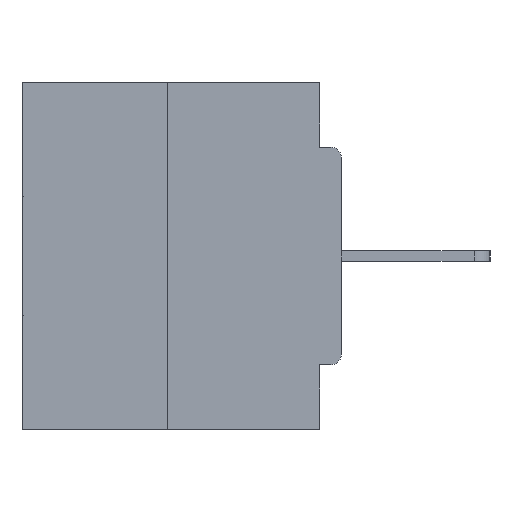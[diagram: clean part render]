
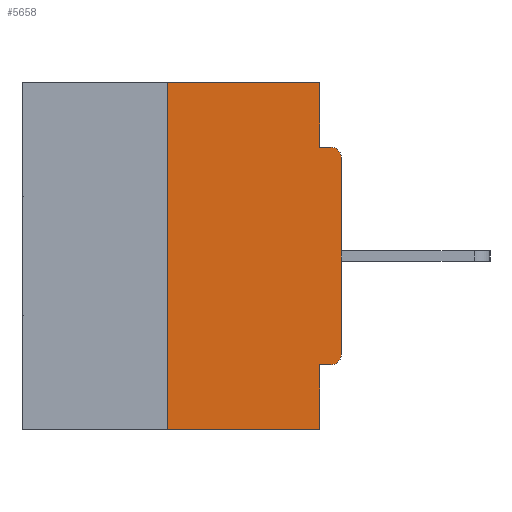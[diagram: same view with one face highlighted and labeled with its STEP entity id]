
A CAD part, left-side view. The second image highlights one B-rep face of the part: STEP entity #5658.
In plain terms, the highlighted planar face has unit normal (-1, 0, 0).
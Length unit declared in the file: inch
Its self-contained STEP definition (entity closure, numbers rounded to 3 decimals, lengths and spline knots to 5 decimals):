
#301 = LINE ( 'NONE', #3106, #26805 ) ;
#2354 = ORIENTED_EDGE ( 'NONE', *, *, #10486, .F. ) ;
#2415 = CARTESIAN_POINT ( 'NONE',  ( 0., 0., -0.4065 ) ) ;
#2515 = EDGE_CURVE ( 'NONE', #10941, #27300, #4757, .T. ) ;
#2608 = DIRECTION ( 'NONE',  ( 0., -1., 0. ) ) ;
#2764 = VECTOR ( 'NONE', #17830, 39.37008 ) ;
#2920 = EDGE_CURVE ( 'NONE', #7568, #13568, #19948, .T. ) ;
#3105 = ORIENTED_EDGE ( 'NONE', *, *, #10581, .F. ) ;
#3106 = CARTESIAN_POINT ( 'NONE',  ( 0., 0.46, 0. ) ) ;
#3801 = LINE ( 'NONE', #24804, #9874 ) ;
#4358 = DIRECTION ( 'NONE',  ( 0., 0., -1. ) ) ;
#4757 = CIRCLE ( 'NONE', #12188, 0.015 ) ;
#5425 = VECTOR ( 'NONE', #16728, 39.37008 ) ;
#5658 = ADVANCED_FACE ( 'NONE', ( #11987 ), #13768, .F. ) ;
#6357 = VECTOR ( 'NONE', #24160, 39.37008 ) ;
#6729 = CARTESIAN_POINT ( 'NONE',  ( 0., 0.015, -0.1085 ) ) ;
#7568 = VERTEX_POINT ( 'NONE', #27094 ) ;
#8507 = ORIENTED_EDGE ( 'NONE', *, *, #2515, .T. ) ;
#9056 = EDGE_CURVE ( 'NONE', #9649, #16005, #301, .T. ) ;
#9332 = DIRECTION ( 'NONE',  ( 0., 0., -1. ) ) ;
#9472 = DIRECTION ( 'NONE',  ( 0., -1., 0. ) ) ;
#9649 = VERTEX_POINT ( 'NONE', #28711 ) ;
#9679 = LINE ( 'NONE', #2415, #2764 ) ;
#9694 = CARTESIAN_POINT ( 'NONE',  ( 0., 0., -0.3915 ) ) ;
#9874 = VECTOR ( 'NONE', #4358, 39.37008 ) ;
#10486 = EDGE_CURVE ( 'NONE', #22350, #28929, #13092, .T. ) ;
#10581 = EDGE_CURVE ( 'NONE', #16005, #22350, #3801, .T. ) ;
#10941 = VERTEX_POINT ( 'NONE', #26113 ) ;
#11171 = CIRCLE ( 'NONE', #15982, 0.015 ) ;
#11987 = FACE_OUTER_BOUND ( 'NONE', #19914, .T. ) ;
#12012 = VERTEX_POINT ( 'NONE', #26157 ) ;
#12188 = AXIS2_PLACEMENT_3D ( 'NONE', #31875, #31736, #31626 ) ;
#12704 = DIRECTION ( 'NONE',  ( 0., 0., -1. ) ) ;
#12757 = LINE ( 'NONE', #19591, #18703 ) ;
#13043 = ORIENTED_EDGE ( 'NONE', *, *, #25138, .F. ) ;
#13092 = LINE ( 'NONE', #19384, #5425 ) ;
#13142 = DIRECTION ( 'NONE',  ( 1., 0., 0. ) ) ;
#13568 = VERTEX_POINT ( 'NONE', #16201 ) ;
#13600 = EDGE_CURVE ( 'NONE', #27300, #22740, #17678, .T. ) ;
#13768 = PLANE ( 'NONE',  #20550 ) ;
#14583 = CARTESIAN_POINT ( 'NONE',  ( 0., 0.46, 0. ) ) ;
#15982 = AXIS2_PLACEMENT_3D ( 'NONE', #6729, #24567, #9332 ) ;
#16005 = VERTEX_POINT ( 'NONE', #16865 ) ;
#16201 = CARTESIAN_POINT ( 'NONE',  ( 0., 0.031, -0.5 ) ) ;
#16315 = CARTESIAN_POINT ( 'NONE',  ( 0., 0., 0. ) ) ;
#16681 = EDGE_CURVE ( 'NONE', #12012, #13568, #12757, .T. ) ;
#16728 = DIRECTION ( 'NONE',  ( 0., -1., 0. ) ) ;
#16865 = CARTESIAN_POINT ( 'NONE',  ( 0., 0.031, 0. ) ) ;
#17678 = LINE ( 'NONE', #16315, #23639 ) ;
#17830 = DIRECTION ( 'NONE',  ( 0., 1., 0. ) ) ;
#18353 = ORIENTED_EDGE ( 'NONE', *, *, #2920, .F. ) ;
#18633 = CARTESIAN_POINT ( 'NONE',  ( 0., 0.031, -0.0935 ) ) ;
#18703 = VECTOR ( 'NONE', #9472, 39.37008 ) ;
#18858 = DIRECTION ( 'NONE',  ( 0., 0., 1. ) ) ;
#19384 = CARTESIAN_POINT ( 'NONE',  ( 0., 0., -0.0935 ) ) ;
#19591 = CARTESIAN_POINT ( 'NONE',  ( 0., 0.46, -0.5 ) ) ;
#19914 = EDGE_LOOP ( 'NONE', ( #30099, #13043, #28129, #18353, #28620, #8507, #23987, #31843, #2354, #3105 ) ) ;
#19948 = LINE ( 'NONE', #24026, #6357 ) ;
#20550 = AXIS2_PLACEMENT_3D ( 'NONE', #14583, #13142, #12704 ) ;
#20634 = VECTOR ( 'NONE', #25137, 39.37008 ) ;
#21402 = CARTESIAN_POINT ( 'NONE',  ( 0., 0.015, -0.0935 ) ) ;
#22350 = VERTEX_POINT ( 'NONE', #18633 ) ;
#22740 = VERTEX_POINT ( 'NONE', #32706 ) ;
#23639 = VECTOR ( 'NONE', #18858, 39.37008 ) ;
#23987 = ORIENTED_EDGE ( 'NONE', *, *, #13600, .T. ) ;
#24026 = CARTESIAN_POINT ( 'NONE',  ( 0., 0.031, -0.5 ) ) ;
#24160 = DIRECTION ( 'NONE',  ( 0., 0., -1. ) ) ;
#24567 = DIRECTION ( 'NONE',  ( -1., 0., 0. ) ) ;
#24804 = CARTESIAN_POINT ( 'NONE',  ( 0., 0.031, 0. ) ) ;
#25137 = DIRECTION ( 'NONE',  ( 0., 0., 1. ) ) ;
#25138 = EDGE_CURVE ( 'NONE', #12012, #9649, #28130, .T. ) ;
#26113 = CARTESIAN_POINT ( 'NONE',  ( 0., 0.015, -0.4065 ) ) ;
#26157 = CARTESIAN_POINT ( 'NONE',  ( 0., 0.25, -0.5 ) ) ;
#26805 = VECTOR ( 'NONE', #2608, 39.37008 ) ;
#27094 = CARTESIAN_POINT ( 'NONE',  ( 0., 0.031, -0.4065 ) ) ;
#27300 = VERTEX_POINT ( 'NONE', #9694 ) ;
#27847 = EDGE_CURVE ( 'NONE', #22740, #28929, #11171, .T. ) ;
#28129 = ORIENTED_EDGE ( 'NONE', *, *, #16681, .T. ) ;
#28130 = LINE ( 'NONE', #32570, #20634 ) ;
#28620 = ORIENTED_EDGE ( 'NONE', *, *, #32126, .F. ) ;
#28711 = CARTESIAN_POINT ( 'NONE',  ( 0., 0.25, 0. ) ) ;
#28929 = VERTEX_POINT ( 'NONE', #21402 ) ;
#30099 = ORIENTED_EDGE ( 'NONE', *, *, #9056, .F. ) ;
#31626 = DIRECTION ( 'NONE',  ( 0., 0., -1. ) ) ;
#31736 = DIRECTION ( 'NONE',  ( -1., 0., 0. ) ) ;
#31843 = ORIENTED_EDGE ( 'NONE', *, *, #27847, .T. ) ;
#31875 = CARTESIAN_POINT ( 'NONE',  ( 0., 0.015, -0.3915 ) ) ;
#32126 = EDGE_CURVE ( 'NONE', #10941, #7568, #9679, .T. ) ;
#32570 = CARTESIAN_POINT ( 'NONE',  ( 0., 0.25, 0. ) ) ;
#32706 = CARTESIAN_POINT ( 'NONE',  ( 0., 0., -0.1085 ) ) ;
